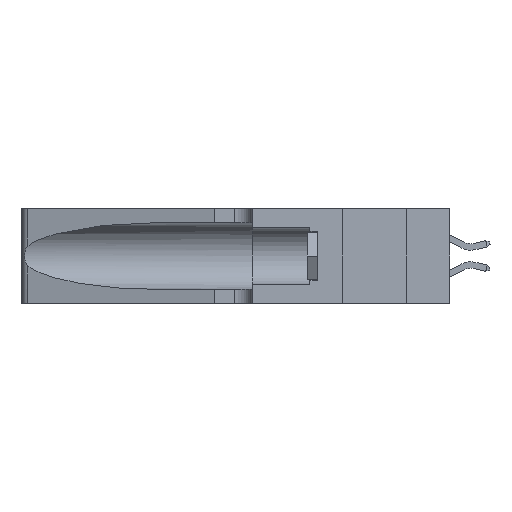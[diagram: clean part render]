
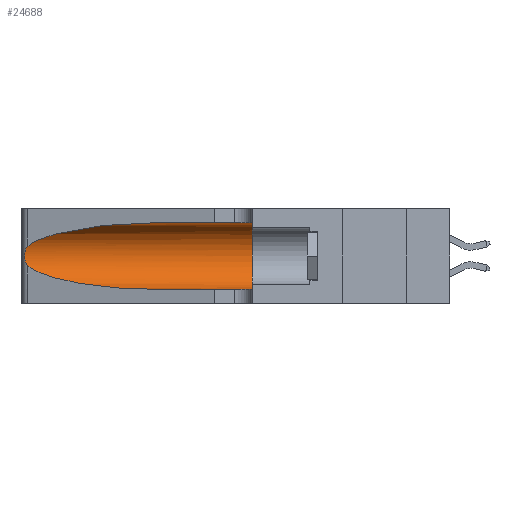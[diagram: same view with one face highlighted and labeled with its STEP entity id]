
A CAD part, left-side view. The second image highlights one B-rep face of the part: STEP entity #24688.
In plain terms, the highlighted cylindrical face has radius 3.308 mm (diameter 6.617 mm), a partial arc.
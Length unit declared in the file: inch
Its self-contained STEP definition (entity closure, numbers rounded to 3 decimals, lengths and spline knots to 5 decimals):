
#15 = CARTESIAN_POINT ( 'NONE',  ( 0.25789, 1.23486, 0.15765 ) ) ;
#537 =( BOUNDED_CURVE ( )  B_SPLINE_CURVE ( 3, ( #22736, #6007, #25525, #8824 ),
 .UNSPECIFIED., .F., .F. ) 
 B_SPLINE_CURVE_WITH_KNOTS ( ( 4, 4 ),
 ( 3.44316, 4.71239 ),
 .UNSPECIFIED. ) 
 CURVE ( )  GEOMETRIC_REPRESENTATION_ITEM ( )  RATIONAL_B_SPLINE_CURVE ( ( 1., 0.87, 0.87, 1. ) ) 
 REPRESENTATION_ITEM ( '' )  );
#816 = ORIENTED_EDGE ( 'NONE', *, *, #4860, .F. ) ;
#1243 = VECTOR ( 'NONE', #28036, 39.37008 ) ;
#2907 = CARTESIAN_POINT ( 'NONE',  ( 0.25555, 1.22993, 0.14849 ) ) ;
#4860 = EDGE_CURVE ( 'NONE', #10000, #9987, #14308, .T. ) ;
#5568 = CARTESIAN_POINT ( 'NONE',  ( 0.1305, 0.35, 0.05475 ) ) ;
#6007 = CARTESIAN_POINT ( 'NONE',  ( 0.2373, 1.15595, 0.08982 ) ) ;
#6165 = CARTESIAN_POINT ( 'NONE',  ( 0.1305, 0.35, 0.31525 ) ) ;
#6856 = VECTOR ( 'NONE', #13826, 39.37008 ) ;
#7014 = VERTEX_POINT ( 'NONE', #12942 ) ;
#8459 = CARTESIAN_POINT ( 'NONE',  ( 0.25787, 1.23484, 0.2124 ) ) ;
#8565 = ORIENTED_EDGE ( 'NONE', *, *, #29659, .F. ) ;
#8577 = EDGE_CURVE ( 'NONE', #7014, #22583, #23621, .T. ) ;
#8824 = CARTESIAN_POINT ( 'NONE',  ( 0.1305, 0.72297, 0.05475 ) ) ;
#9073 = CARTESIAN_POINT ( 'NONE',  ( 0.25487, 1.22718, 0.14631 ) ) ;
#9608 = VERTEX_POINT ( 'NONE', #21048 ) ;
#9987 = VERTEX_POINT ( 'NONE', #6165 ) ;
#10000 = VERTEX_POINT ( 'NONE', #31204 ) ;
#10980 = ORIENTED_EDGE ( 'NONE', *, *, #34725, .T. ) ;
#11273 = CARTESIAN_POINT ( 'NONE',  ( 0.26018, 1.23835, 0.19895 ) ) ;
#12189 = DIRECTION ( 'NONE',  ( 0., -1., 0. ) ) ;
#12942 = CARTESIAN_POINT ( 'NONE',  ( 0.1305, 0.72297, 0.05475 ) ) ;
#13070 = AXIS2_PLACEMENT_3D ( 'NONE', #30974, #14365, #33774 ) ;
#13490 = CARTESIAN_POINT ( 'NONE',  ( 0.18966, 0.96281, 0.31525 ) ) ;
#13826 = DIRECTION ( 'NONE',  ( 0., -1., 0. ) ) ;
#14076 = CARTESIAN_POINT ( 'NONE',  ( 0.26075, 1.23896, 0.178 ) ) ;
#14308 = LINE ( 'NONE', #27672, #6856 ) ;
#14365 = DIRECTION ( 'NONE',  ( 0., 1., 0. ) ) ;
#14745 =( BOUNDED_CURVE ( )  B_SPLINE_CURVE ( 3, ( #27346, #13490, #32885, #16278 ),
 .UNSPECIFIED., .F., .T. ) 
 B_SPLINE_CURVE_WITH_KNOTS ( ( 4, 4 ),
 ( 1.5708, 2.84003 ),
 .UNSPECIFIED. ) 
 CURVE ( )  GEOMETRIC_REPRESENTATION_ITEM ( )  RATIONAL_B_SPLINE_CURVE ( ( 1., 0.87, 0.87, 1. ) ) 
 REPRESENTATION_ITEM ( '' )  );
#15035 = VERTEX_POINT ( 'NONE', #9073 ) ;
#15095 = CYLINDRICAL_SURFACE ( 'NONE', #19742, 0.13025 ) ;
#15096 = ORIENTED_EDGE ( 'NONE', *, *, #8577, .T. ) ;
#15496 = EDGE_CURVE ( 'NONE', #9608, #15035, #26590, .T. ) ;
#16002 = FACE_OUTER_BOUND ( 'NONE', #22621, .T. ) ;
#16278 = CARTESIAN_POINT ( 'NONE',  ( 0.25487, 1.22718, 0.22369 ) ) ;
#16749 = CARTESIAN_POINT ( 'NONE',  ( 0.25555, 1.22994, 0.2215 ) ) ;
#16861 = CARTESIAN_POINT ( 'NONE',  ( 0.25856, 1.23593, 0.16098 ) ) ;
#19680 = CARTESIAN_POINT ( 'NONE',  ( 0.25639, 1.23186, 0.15144 ) ) ;
#19742 = AXIS2_PLACEMENT_3D ( 'NONE', #28825, #12189, #31602 ) ;
#20459 = EDGE_CURVE ( 'NONE', #15035, #7014, #537, .T. ) ;
#21048 = CARTESIAN_POINT ( 'NONE',  ( 0.25487, 1.22718, 0.22369 ) ) ;
#22361 = CARTESIAN_POINT ( 'NONE',  ( 0.25487, 1.22718, 0.22369 ) ) ;
#22478 = CARTESIAN_POINT ( 'NONE',  ( 0.1305, 1.61858, 0.05475 ) ) ;
#22482 = CARTESIAN_POINT ( 'NONE',  ( 0.25487, 1.22718, 0.14631 ) ) ;
#22583 = VERTEX_POINT ( 'NONE', #5568 ) ;
#22621 = EDGE_LOOP ( 'NONE', ( #10980, #23021, #23852, #15096, #8565, #816 ) ) ;
#22736 = CARTESIAN_POINT ( 'NONE',  ( 0.25487, 1.22718, 0.14631 ) ) ;
#23021 = ORIENTED_EDGE ( 'NONE', *, *, #15496, .T. ) ;
#23621 = LINE ( 'NONE', #22478, #1243 ) ;
#23852 = ORIENTED_EDGE ( 'NONE', *, *, #20459, .T. ) ;
#24688 = ADVANCED_FACE ( 'NONE', ( #16002 ), #15095, .F. ) ;
#25171 = CARTESIAN_POINT ( 'NONE',  ( 0.25639, 1.23184, 0.21858 ) ) ;
#25525 = CARTESIAN_POINT ( 'NONE',  ( 0.18966, 0.96281, 0.05475 ) ) ;
#26590 = B_SPLINE_CURVE_WITH_KNOTS ( 'NONE', 3,
 ( #22361, #16749, #25171, #8459, #27925, #11273, #30687, #14076, #33485, #16861, #15, #19680, #2907, #22482 ),
 .UNSPECIFIED., .F., .F.,
 ( 4, 2, 2, 2, 2, 2, 4 ),
 ( 0., 0.00027, 0.00053, 0.00107, 0.0016, 0.00187, 0.00214 ),
 .UNSPECIFIED. ) ;
#27298 = CIRCLE ( 'NONE', #13070, 0.13025 ) ;
#27346 = CARTESIAN_POINT ( 'NONE',  ( 0.1305, 0.72297, 0.31525 ) ) ;
#27672 = CARTESIAN_POINT ( 'NONE',  ( 0.1305, 1.61858, 0.31525 ) ) ;
#27925 = CARTESIAN_POINT ( 'NONE',  ( 0.25854, 1.2359, 0.20912 ) ) ;
#28036 = DIRECTION ( 'NONE',  ( 0., -1., 0. ) ) ;
#28825 = CARTESIAN_POINT ( 'NONE',  ( 0.1305, 1.61858, 0.185 ) ) ;
#29659 = EDGE_CURVE ( 'NONE', #9987, #22583, #27298, .T. ) ;
#30687 = CARTESIAN_POINT ( 'NONE',  ( 0.26075, 1.23896, 0.19203 ) ) ;
#30974 = CARTESIAN_POINT ( 'NONE',  ( 0.1305, 0.35, 0.185 ) ) ;
#31204 = CARTESIAN_POINT ( 'NONE',  ( 0.1305, 0.72297, 0.31525 ) ) ;
#31602 = DIRECTION ( 'NONE',  ( 0., 0., -1. ) ) ;
#32885 = CARTESIAN_POINT ( 'NONE',  ( 0.2373, 1.15595, 0.28018 ) ) ;
#33485 = CARTESIAN_POINT ( 'NONE',  ( 0.26017, 1.23833, 0.17102 ) ) ;
#33774 = DIRECTION ( 'NONE',  ( 0., 0., 1. ) ) ;
#34725 = EDGE_CURVE ( 'NONE', #10000, #9608, #14745, .T. ) ;
